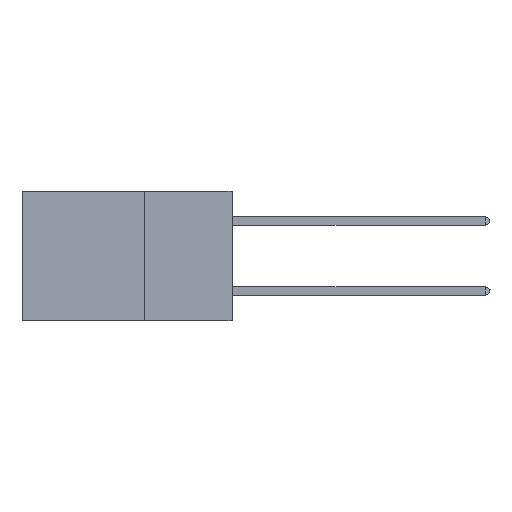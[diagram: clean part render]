
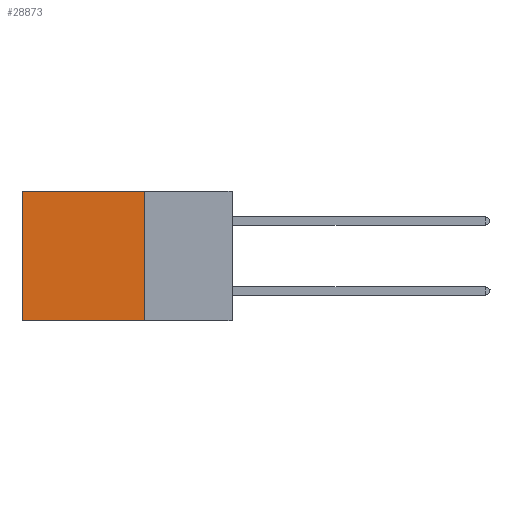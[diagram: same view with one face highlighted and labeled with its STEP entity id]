
A CAD part, left-side view. The second image highlights one B-rep face of the part: STEP entity #28873.
In plain terms, the highlighted planar face has unit normal (-1, 0, 0).
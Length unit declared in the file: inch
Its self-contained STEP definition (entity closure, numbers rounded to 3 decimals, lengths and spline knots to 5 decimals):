
#1273 = EDGE_CURVE ( 'NONE', #6933, #31159, #27784, .T. ) ;
#1678 = CARTESIAN_POINT ( 'NONE',  ( 0.2875, 0.25, 0. ) ) ;
#2208 = LINE ( 'NONE', #29453, #31706 ) ;
#2407 = VECTOR ( 'NONE', #7436, 39.37008 ) ;
#2546 = VECTOR ( 'NONE', #5128, 39.37008 ) ;
#5128 = DIRECTION ( 'NONE',  ( 0., 1., 0. ) ) ;
#5875 = DIRECTION ( 'NONE',  ( 1., 0., 0. ) ) ;
#6933 = VERTEX_POINT ( 'NONE', #26931 ) ;
#7436 = DIRECTION ( 'NONE',  ( 0., 1., 0. ) ) ;
#7970 = DIRECTION ( 'NONE',  ( 0., 0., -1. ) ) ;
#9382 = CARTESIAN_POINT ( 'NONE',  ( 0.2875, 0.6, 0. ) ) ;
#9572 = CARTESIAN_POINT ( 'NONE',  ( 0.2875, 0.6, -0.37 ) ) ;
#9866 = ORIENTED_EDGE ( 'NONE', *, *, #1273, .F. ) ;
#11972 = AXIS2_PLACEMENT_3D ( 'NONE', #29568, #5875, #16529 ) ;
#12329 = LINE ( 'NONE', #1678, #2407 ) ;
#13802 = CARTESIAN_POINT ( 'NONE',  ( 0.2875, 0.25, -0.37 ) ) ;
#14178 = DIRECTION ( 'NONE',  ( 0., 0., -1. ) ) ;
#15730 = VECTOR ( 'NONE', #14178, 39.37008 ) ;
#15866 = VERTEX_POINT ( 'NONE', #9382 ) ;
#16529 = DIRECTION ( 'NONE',  ( 0., 0., -1. ) ) ;
#16567 = EDGE_CURVE ( 'NONE', #31159, #32610, #21197, .T. ) ;
#20384 = EDGE_CURVE ( 'NONE', #15866, #32610, #2208, .T. ) ;
#21197 = LINE ( 'NONE', #32368, #2546 ) ;
#21476 = ORIENTED_EDGE ( 'NONE', *, *, #27297, .T. ) ;
#21767 = FACE_OUTER_BOUND ( 'NONE', #25251, .T. ) ;
#24840 = ORIENTED_EDGE ( 'NONE', *, *, #20384, .T. ) ;
#25251 = EDGE_LOOP ( 'NONE', ( #24840, #33869, #9866, #21476 ) ) ;
#26931 = CARTESIAN_POINT ( 'NONE',  ( 0.2875, 0.25, 0. ) ) ;
#27297 = EDGE_CURVE ( 'NONE', #6933, #15866, #12329, .T. ) ;
#27784 = LINE ( 'NONE', #30573, #15730 ) ;
#28873 = ADVANCED_FACE ( 'NONE', ( #21767 ), #32415, .F. ) ;
#29453 = CARTESIAN_POINT ( 'NONE',  ( 0.2875, 0.6, 0. ) ) ;
#29568 = CARTESIAN_POINT ( 'NONE',  ( 0.2875, 0.25, 0. ) ) ;
#30573 = CARTESIAN_POINT ( 'NONE',  ( 0.2875, 0.25, 0. ) ) ;
#31159 = VERTEX_POINT ( 'NONE', #13802 ) ;
#31706 = VECTOR ( 'NONE', #7970, 39.37008 ) ;
#32368 = CARTESIAN_POINT ( 'NONE',  ( 0.2875, 0.25, -0.37 ) ) ;
#32415 = PLANE ( 'NONE',  #11972 ) ;
#32610 = VERTEX_POINT ( 'NONE', #9572 ) ;
#33869 = ORIENTED_EDGE ( 'NONE', *, *, #16567, .F. ) ;
